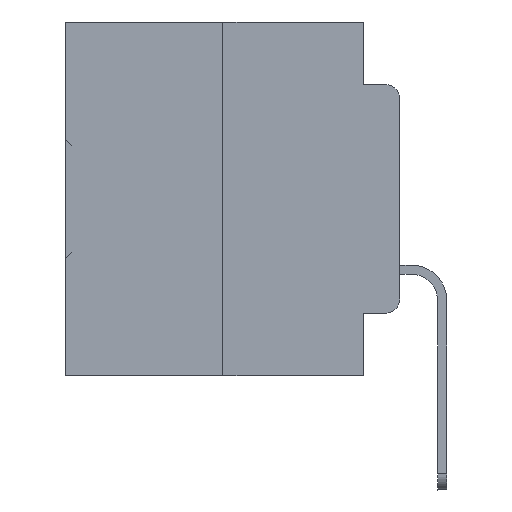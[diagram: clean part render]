
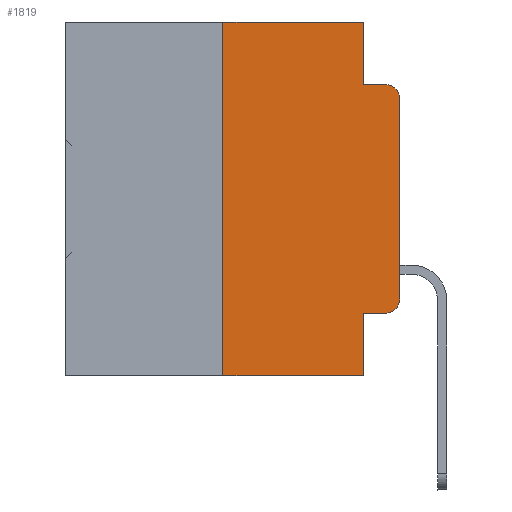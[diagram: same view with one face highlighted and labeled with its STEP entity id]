
A CAD part, left-side view. The second image highlights one B-rep face of the part: STEP entity #1819.
In plain terms, the highlighted planar face has unit normal (-1, 0, 0).
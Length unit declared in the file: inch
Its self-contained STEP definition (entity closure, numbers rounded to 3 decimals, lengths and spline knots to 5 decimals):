
#212 = LINE ( 'NONE', #28250, #32935 ) ;
#411 = CARTESIAN_POINT ( 'NONE',  ( 0., 0.051, 0. ) ) ;
#503 = ORIENTED_EDGE ( 'NONE', *, *, #4076, .F. ) ;
#1484 = VERTEX_POINT ( 'NONE', #11402 ) ;
#1702 = EDGE_CURVE ( 'NONE', #14551, #3713, #12310, .T. ) ;
#1707 = CIRCLE ( 'NONE', #6321, 0.02 ) ;
#1732 = ORIENTED_EDGE ( 'NONE', *, *, #22728, .T. ) ;
#1819 = ADVANCED_FACE ( 'NONE', ( #32587 ), #35317, .F. ) ;
#2017 = ORIENTED_EDGE ( 'NONE', *, *, #25239, .T. ) ;
#2040 = AXIS2_PLACEMENT_3D ( 'NONE', #18445, #10509, #13204 ) ;
#2548 = ORIENTED_EDGE ( 'NONE', *, *, #10723, .F. ) ;
#2768 = LINE ( 'NONE', #19791, #33295 ) ;
#2912 = EDGE_CURVE ( 'NONE', #26418, #8216, #8703, .T. ) ;
#3052 = EDGE_LOOP ( 'NONE', ( #31258, #2017, #18906, #16502, #503, #2548, #30659, #24107, #3251, #1732 ) ) ;
#3251 = ORIENTED_EDGE ( 'NONE', *, *, #2912, .T. ) ;
#3506 = VECTOR ( 'NONE', #20952, 39.37008 ) ;
#3713 = VERTEX_POINT ( 'NONE', #19827 ) ;
#4076 = EDGE_CURVE ( 'NONE', #10016, #9981, #2768, .T. ) ;
#4211 = EDGE_CURVE ( 'NONE', #9981, #14551, #16359, .T. ) ;
#4730 = CARTESIAN_POINT ( 'NONE',  ( 0., 0.051, -0.5 ) ) ;
#4767 = VERTEX_POINT ( 'NONE', #4730 ) ;
#5172 = EDGE_CURVE ( 'NONE', #24918, #1484, #13369, .T. ) ;
#5506 = CARTESIAN_POINT ( 'NONE',  ( 0., 0.02, -0.3915 ) ) ;
#5810 = EDGE_CURVE ( 'NONE', #26418, #4767, #212, .T. ) ;
#6321 = AXIS2_PLACEMENT_3D ( 'NONE', #5506, #27951, #14188 ) ;
#7593 = CARTESIAN_POINT ( 'NONE',  ( 0., 0.25, 0. ) ) ;
#7646 = LINE ( 'NONE', #32620, #11028 ) ;
#8216 = VERTEX_POINT ( 'NONE', #24366 ) ;
#8703 = LINE ( 'NONE', #31131, #34421 ) ;
#9981 = VERTEX_POINT ( 'NONE', #10498 ) ;
#10016 = VERTEX_POINT ( 'NONE', #7593 ) ;
#10498 = CARTESIAN_POINT ( 'NONE',  ( 0., 0.051, 0. ) ) ;
#10509 = DIRECTION ( 'NONE',  ( 1., 0., 0. ) ) ;
#10723 = EDGE_CURVE ( 'NONE', #20281, #10016, #7646, .T. ) ;
#11028 = VECTOR ( 'NONE', #21886, 39.37008 ) ;
#11402 = CARTESIAN_POINT ( 'NONE',  ( 0., 0., -0.1085 ) ) ;
#11421 = DIRECTION ( 'NONE',  ( 0., 0., -1. ) ) ;
#12145 = CARTESIAN_POINT ( 'NONE',  ( 0., 0.051, -0.4115 ) ) ;
#12310 = LINE ( 'NONE', #23703, #19382 ) ;
#12472 = DIRECTION ( 'NONE',  ( 0., -1., 0. ) ) ;
#12645 = VECTOR ( 'NONE', #12472, 39.37008 ) ;
#13204 = DIRECTION ( 'NONE',  ( 0., 0., -1. ) ) ;
#13369 = LINE ( 'NONE', #24020, #3506 ) ;
#14188 = DIRECTION ( 'NONE',  ( 0., 0., -1. ) ) ;
#14291 = DIRECTION ( 'NONE',  ( 0., -1., 0. ) ) ;
#14551 = VERTEX_POINT ( 'NONE', #15195 ) ;
#15195 = CARTESIAN_POINT ( 'NONE',  ( 0., 0.051, -0.0885 ) ) ;
#16359 = LINE ( 'NONE', #411, #22880 ) ;
#16366 = EDGE_CURVE ( 'NONE', #20281, #4767, #21146, .T. ) ;
#16502 = ORIENTED_EDGE ( 'NONE', *, *, #4211, .F. ) ;
#18445 = CARTESIAN_POINT ( 'NONE',  ( 0., 0.473, 0. ) ) ;
#18578 = AXIS2_PLACEMENT_3D ( 'NONE', #23345, #34049, #25700 ) ;
#18906 = ORIENTED_EDGE ( 'NONE', *, *, #1702, .F. ) ;
#19382 = VECTOR ( 'NONE', #23506, 39.37008 ) ;
#19791 = CARTESIAN_POINT ( 'NONE',  ( 0., 0.473, 0. ) ) ;
#19827 = CARTESIAN_POINT ( 'NONE',  ( 0., 0.02, -0.0885 ) ) ;
#20281 = VERTEX_POINT ( 'NONE', #35073 ) ;
#20952 = DIRECTION ( 'NONE',  ( 0., 0., 1. ) ) ;
#21146 = LINE ( 'NONE', #26406, #12645 ) ;
#21886 = DIRECTION ( 'NONE',  ( 0., 0., 1. ) ) ;
#22728 = EDGE_CURVE ( 'NONE', #8216, #24918, #1707, .T. ) ;
#22880 = VECTOR ( 'NONE', #28103, 39.37008 ) ;
#23345 = CARTESIAN_POINT ( 'NONE',  ( 0., 0.02, -0.1085 ) ) ;
#23506 = DIRECTION ( 'NONE',  ( 0., -1., 0. ) ) ;
#23703 = CARTESIAN_POINT ( 'NONE',  ( 0., 0.051, -0.0885 ) ) ;
#24020 = CARTESIAN_POINT ( 'NONE',  ( 0., 0., 0. ) ) ;
#24107 = ORIENTED_EDGE ( 'NONE', *, *, #5810, .F. ) ;
#24366 = CARTESIAN_POINT ( 'NONE',  ( 0., 0.02, -0.4115 ) ) ;
#24918 = VERTEX_POINT ( 'NONE', #26670 ) ;
#24920 = CIRCLE ( 'NONE', #18578, 0.02 ) ;
#25239 = EDGE_CURVE ( 'NONE', #1484, #3713, #24920, .T. ) ;
#25700 = DIRECTION ( 'NONE',  ( 0., 0., -1. ) ) ;
#26406 = CARTESIAN_POINT ( 'NONE',  ( 0., 0.473, -0.5 ) ) ;
#26418 = VERTEX_POINT ( 'NONE', #12145 ) ;
#26670 = CARTESIAN_POINT ( 'NONE',  ( 0., 0., -0.3915 ) ) ;
#27951 = DIRECTION ( 'NONE',  ( -1., 0., 0. ) ) ;
#28103 = DIRECTION ( 'NONE',  ( 0., 0., -1. ) ) ;
#28250 = CARTESIAN_POINT ( 'NONE',  ( 0., 0.051, 0. ) ) ;
#30659 = ORIENTED_EDGE ( 'NONE', *, *, #16366, .T. ) ;
#31131 = CARTESIAN_POINT ( 'NONE',  ( 0., 0.051, -0.4115 ) ) ;
#31258 = ORIENTED_EDGE ( 'NONE', *, *, #5172, .T. ) ;
#32587 = FACE_OUTER_BOUND ( 'NONE', #3052, .T. ) ;
#32620 = CARTESIAN_POINT ( 'NONE',  ( 0., 0.25, 0. ) ) ;
#32935 = VECTOR ( 'NONE', #11421, 39.37008 ) ;
#33295 = VECTOR ( 'NONE', #35734, 39.37008 ) ;
#34049 = DIRECTION ( 'NONE',  ( -1., 0., 0. ) ) ;
#34421 = VECTOR ( 'NONE', #14291, 39.37008 ) ;
#35073 = CARTESIAN_POINT ( 'NONE',  ( 0., 0.25, -0.5 ) ) ;
#35317 = PLANE ( 'NONE',  #2040 ) ;
#35734 = DIRECTION ( 'NONE',  ( 0., -1., 0. ) ) ;
